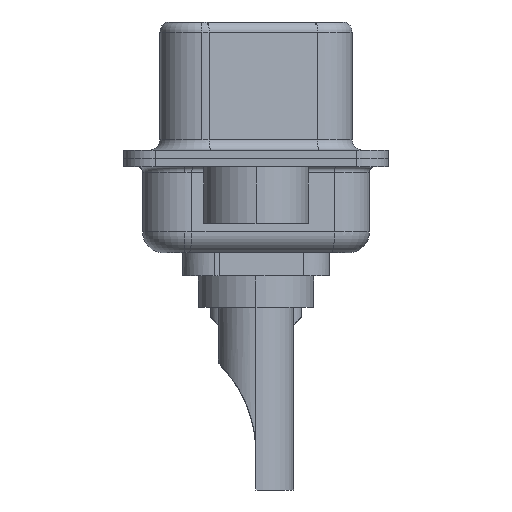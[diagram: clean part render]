
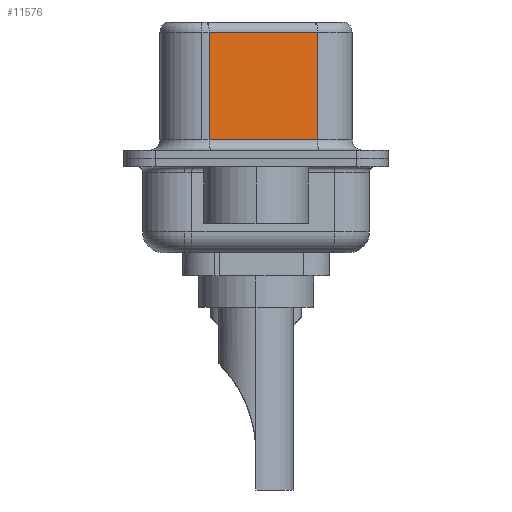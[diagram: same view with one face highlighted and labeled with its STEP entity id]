
A CAD part, left-side view. The second image highlights one B-rep face of the part: STEP entity #11576.
In plain terms, the highlighted planar face has unit normal (-0.985, -0.174, 0).
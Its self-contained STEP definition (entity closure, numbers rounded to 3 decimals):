
#889 = CARTESIAN_POINT ( 'NONE',  ( 4.58, -2.927, 6.52 ) ) ;
#1294 = CARTESIAN_POINT ( 'NONE',  ( 4.58, -2.927, 0.9 ) ) ;
#1391 = CARTESIAN_POINT ( 'NONE',  ( 4.58, -2.927, 6.02 ) ) ;
#2100 = CARTESIAN_POINT ( 'NONE',  ( 3.67, 2.233, 0.9 ) ) ;
#2287 = VECTOR ( 'NONE', #9866, 1000. ) ;
#2442 = LINE ( 'NONE', #10822, #6373 ) ;
#2459 = CARTESIAN_POINT ( 'NONE',  ( 4.58, -2.927, 6.02 ) ) ;
#3243 = LINE ( 'NONE', #13717, #20678 ) ;
#3705 = DIRECTION ( 'NONE',  ( 0., 0., -1. ) ) ;
#3751 = VERTEX_POINT ( 'NONE', #2100 ) ;
#3898 = VERTEX_POINT ( 'NONE', #5221 ) ;
#4260 = PLANE ( 'NONE',  #4992 ) ;
#4332 = EDGE_LOOP ( 'NONE', ( #16384, #18221, #16376, #9400 ) ) ;
#4992 = AXIS2_PLACEMENT_3D ( 'NONE', #889, #19448, #9316 ) ;
#5221 = CARTESIAN_POINT ( 'NONE',  ( 3.67, 2.233, 6.02 ) ) ;
#6373 = VECTOR ( 'NONE', #20970, 1000. ) ;
#7319 = VERTEX_POINT ( 'NONE', #1294 ) ;
#8111 = EDGE_CURVE ( 'NONE', #14814, #7319, #3243, .T. ) ;
#9316 = DIRECTION ( 'NONE',  ( -0.174, 0.985, 0. ) ) ;
#9400 = ORIENTED_EDGE ( 'NONE', *, *, #15454, .T. ) ;
#9527 = LINE ( 'NONE', #1391, #10075 ) ;
#9747 = DIRECTION ( 'NONE',  ( -0.174, 0.985, 0. ) ) ;
#9866 = DIRECTION ( 'NONE',  ( 0., 0., -1. ) ) ;
#10075 = VECTOR ( 'NONE', #9747, 1000. ) ;
#10822 = CARTESIAN_POINT ( 'NONE',  ( 4.58, -2.927, 0.9 ) ) ;
#11226 = LINE ( 'NONE', #16551, #2287 ) ;
#11560 = FACE_OUTER_BOUND ( 'NONE', #4332, .T. ) ;
#11576 = ADVANCED_FACE ( 'NONE', ( #11560 ), #4260, .F. ) ;
#13717 = CARTESIAN_POINT ( 'NONE',  ( 4.58, -2.927, 6.52 ) ) ;
#14814 = VERTEX_POINT ( 'NONE', #2459 ) ;
#15454 = EDGE_CURVE ( 'NONE', #3751, #7319, #2442, .T. ) ;
#16376 = ORIENTED_EDGE ( 'NONE', *, *, #20614, .T. ) ;
#16384 = ORIENTED_EDGE ( 'NONE', *, *, #8111, .F. ) ;
#16551 = CARTESIAN_POINT ( 'NONE',  ( 3.67, 2.233, 6.52 ) ) ;
#16698 = EDGE_CURVE ( 'NONE', #14814, #3898, #9527, .T. ) ;
#18221 = ORIENTED_EDGE ( 'NONE', *, *, #16698, .T. ) ;
#19448 = DIRECTION ( 'NONE',  ( 0.985, 0.174, 0. ) ) ;
#20614 = EDGE_CURVE ( 'NONE', #3898, #3751, #11226, .T. ) ;
#20678 = VECTOR ( 'NONE', #3705, 1000. ) ;
#20970 = DIRECTION ( 'NONE',  ( 0.174, -0.985, 0. ) ) ;
